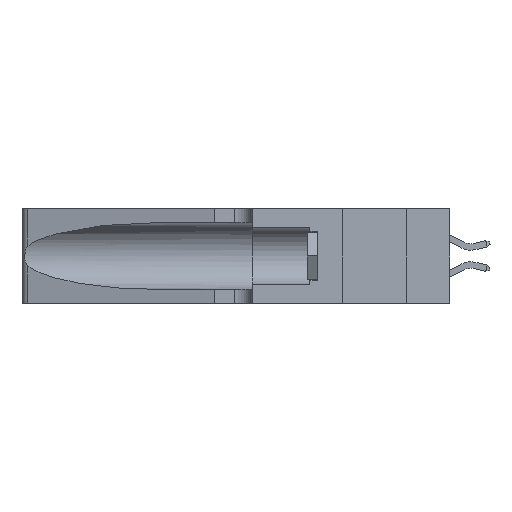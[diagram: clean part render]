
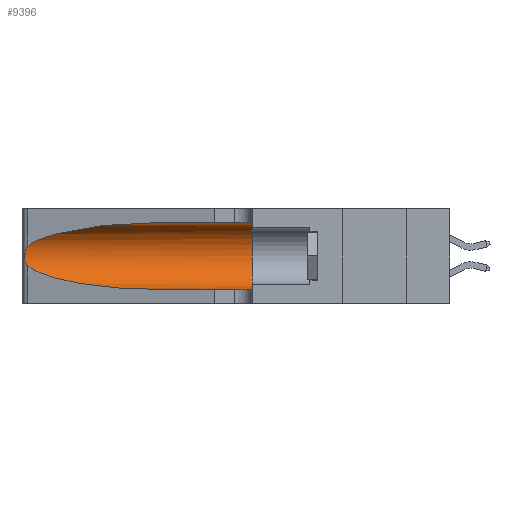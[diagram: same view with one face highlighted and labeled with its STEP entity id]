
A CAD part, left-side view. The second image highlights one B-rep face of the part: STEP entity #9396.
In plain terms, the highlighted cylindrical face has radius 3.308 mm (diameter 6.617 mm), a partial arc.
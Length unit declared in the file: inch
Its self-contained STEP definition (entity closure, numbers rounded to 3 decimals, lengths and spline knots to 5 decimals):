
#373 = CARTESIAN_POINT ( 'NONE',  ( 0.25487, 1.22718, 0.22369 ) ) ;
#752 = CARTESIAN_POINT ( 'NONE',  ( 0.18966, 0.96281, 0.05475 ) ) ;
#1265 =( BOUNDED_CURVE ( )  B_SPLINE_CURVE ( 3, ( #36432, #39600, #8391, #30260 ),
 .UNSPECIFIED., .F., .F. ) 
 B_SPLINE_CURVE_WITH_KNOTS ( ( 4, 4 ),
 ( 1.5708, 2.84003 ),
 .UNSPECIFIED. ) 
 CURVE ( )  GEOMETRIC_REPRESENTATION_ITEM ( )  RATIONAL_B_SPLINE_CURVE ( ( 1., 0.87, 0.87, 1. ) ) 
 REPRESENTATION_ITEM ( '' )  );
#2405 = VERTEX_POINT ( 'NONE', #38991 ) ;
#2751 = CARTESIAN_POINT ( 'NONE',  ( 0.26075, 1.23896, 0.178 ) ) ;
#2760 = VECTOR ( 'NONE', #14665, 39.37008 ) ;
#3657 = VERTEX_POINT ( 'NONE', #31638 ) ;
#3982 = VERTEX_POINT ( 'NONE', #23694 ) ;
#4009 = DIRECTION ( 'NONE',  ( 0., -1., 0. ) ) ;
#4351 = ORIENTED_EDGE ( 'NONE', *, *, #28018, .T. ) ;
#5039 = AXIS2_PLACEMENT_3D ( 'NONE', #30613, #11892, #33789 ) ;
#5984 = CARTESIAN_POINT ( 'NONE',  ( 0.25856, 1.23593, 0.16098 ) ) ;
#6492 = ORIENTED_EDGE ( 'NONE', *, *, #14828, .F. ) ;
#6604 = FACE_OUTER_BOUND ( 'NONE', #36968, .T. ) ;
#7046 = CARTESIAN_POINT ( 'NONE',  ( 0.2373, 1.15595, 0.08982 ) ) ;
#7260 = CARTESIAN_POINT ( 'NONE',  ( 0.1305, 1.61858, 0.185 ) ) ;
#7661 = ORIENTED_EDGE ( 'NONE', *, *, #28254, .T. ) ;
#8391 = CARTESIAN_POINT ( 'NONE',  ( 0.2373, 1.15595, 0.28018 ) ) ;
#8997 = CARTESIAN_POINT ( 'NONE',  ( 0.25487, 1.22718, 0.22369 ) ) ;
#9134 = CARTESIAN_POINT ( 'NONE',  ( 0.25639, 1.23186, 0.15144 ) ) ;
#9387 = CIRCLE ( 'NONE', #5039, 0.13025 ) ;
#9396 = ADVANCED_FACE ( 'NONE', ( #6604 ), #13944, .F. ) ;
#10197 = DIRECTION ( 'NONE',  ( 0., -1., 0. ) ) ;
#10382 = DIRECTION ( 'NONE',  ( 0., 0., -1. ) ) ;
#11090 = EDGE_CURVE ( 'NONE', #3982, #3657, #9387, .T. ) ;
#11173 = LINE ( 'NONE', #14266, #2760 ) ;
#11845 = VERTEX_POINT ( 'NONE', #34299 ) ;
#11892 = DIRECTION ( 'NONE',  ( 0., 1., 0. ) ) ;
#12264 = CARTESIAN_POINT ( 'NONE',  ( 0.25487, 1.22718, 0.14631 ) ) ;
#13944 = CYLINDRICAL_SURFACE ( 'NONE', #27838, 0.13025 ) ;
#14266 = CARTESIAN_POINT ( 'NONE',  ( 0.1305, 1.61858, 0.31525 ) ) ;
#14665 = DIRECTION ( 'NONE',  ( 0., -1., 0. ) ) ;
#14828 = EDGE_CURVE ( 'NONE', #2405, #3982, #11173, .T. ) ;
#15176 = VECTOR ( 'NONE', #10197, 39.37008 ) ;
#15287 = CARTESIAN_POINT ( 'NONE',  ( 0.25639, 1.23184, 0.21858 ) ) ;
#15944 =( BOUNDED_CURVE ( )  B_SPLINE_CURVE ( 3, ( #35210, #7046, #752, #22762 ),
 .UNSPECIFIED., .F., .T. ) 
 B_SPLINE_CURVE_WITH_KNOTS ( ( 4, 4 ),
 ( 3.44316, 4.71239 ),
 .UNSPECIFIED. ) 
 CURVE ( )  GEOMETRIC_REPRESENTATION_ITEM ( )  RATIONAL_B_SPLINE_CURVE ( ( 1., 0.87, 0.87, 1. ) ) 
 REPRESENTATION_ITEM ( '' )  );
#16809 = ORIENTED_EDGE ( 'NONE', *, *, #11090, .F. ) ;
#18411 = CARTESIAN_POINT ( 'NONE',  ( 0.25854, 1.2359, 0.20912 ) ) ;
#20166 = B_SPLINE_CURVE_WITH_KNOTS ( 'NONE', 3,
 ( #8997, #33899, #15287, #37200, #18411, #40346, #21565, #2751, #24719, #5984, #27876, #9134, #30989, #12264 ),
 .UNSPECIFIED., .F., .F.,
 ( 4, 2, 2, 2, 2, 2, 4 ),
 ( 0., 0.00027, 0.00053, 0.00107, 0.0016, 0.00187, 0.00214 ),
 .UNSPECIFIED. ) ;
#20733 = VERTEX_POINT ( 'NONE', #21870 ) ;
#21565 = CARTESIAN_POINT ( 'NONE',  ( 0.26075, 1.23896, 0.19203 ) ) ;
#21870 = CARTESIAN_POINT ( 'NONE',  ( 0.1305, 0.72297, 0.05475 ) ) ;
#22762 = CARTESIAN_POINT ( 'NONE',  ( 0.1305, 0.72297, 0.05475 ) ) ;
#23694 = CARTESIAN_POINT ( 'NONE',  ( 0.1305, 0.35, 0.31525 ) ) ;
#24719 = CARTESIAN_POINT ( 'NONE',  ( 0.26017, 1.23833, 0.17102 ) ) ;
#26783 = VERTEX_POINT ( 'NONE', #373 ) ;
#27407 = ORIENTED_EDGE ( 'NONE', *, *, #35561, .T. ) ;
#27838 = AXIS2_PLACEMENT_3D ( 'NONE', #7260, #4009, #10382 ) ;
#27876 = CARTESIAN_POINT ( 'NONE',  ( 0.25789, 1.23486, 0.15765 ) ) ;
#28018 = EDGE_CURVE ( 'NONE', #11845, #20733, #15944, .T. ) ;
#28254 = EDGE_CURVE ( 'NONE', #2405, #26783, #1265, .T. ) ;
#28414 = ORIENTED_EDGE ( 'NONE', *, *, #36589, .T. ) ;
#30260 = CARTESIAN_POINT ( 'NONE',  ( 0.25487, 1.22718, 0.22369 ) ) ;
#30613 = CARTESIAN_POINT ( 'NONE',  ( 0.1305, 0.35, 0.185 ) ) ;
#30989 = CARTESIAN_POINT ( 'NONE',  ( 0.25555, 1.22993, 0.14849 ) ) ;
#31638 = CARTESIAN_POINT ( 'NONE',  ( 0.1305, 0.35, 0.05475 ) ) ;
#33789 = DIRECTION ( 'NONE',  ( 0., 0., 1. ) ) ;
#33899 = CARTESIAN_POINT ( 'NONE',  ( 0.25555, 1.22994, 0.2215 ) ) ;
#34299 = CARTESIAN_POINT ( 'NONE',  ( 0.25487, 1.22718, 0.14631 ) ) ;
#35210 = CARTESIAN_POINT ( 'NONE',  ( 0.25487, 1.22718, 0.14631 ) ) ;
#35561 = EDGE_CURVE ( 'NONE', #20733, #3657, #40168, .T. ) ;
#36432 = CARTESIAN_POINT ( 'NONE',  ( 0.1305, 0.72297, 0.31525 ) ) ;
#36589 = EDGE_CURVE ( 'NONE', #26783, #11845, #20166, .T. ) ;
#36968 = EDGE_LOOP ( 'NONE', ( #7661, #28414, #4351, #27407, #16809, #6492 ) ) ;
#37200 = CARTESIAN_POINT ( 'NONE',  ( 0.25787, 1.23484, 0.2124 ) ) ;
#38260 = CARTESIAN_POINT ( 'NONE',  ( 0.1305, 1.61858, 0.05475 ) ) ;
#38991 = CARTESIAN_POINT ( 'NONE',  ( 0.1305, 0.72297, 0.31525 ) ) ;
#39600 = CARTESIAN_POINT ( 'NONE',  ( 0.18966, 0.96281, 0.31525 ) ) ;
#40168 = LINE ( 'NONE', #38260, #15176 ) ;
#40346 = CARTESIAN_POINT ( 'NONE',  ( 0.26018, 1.23835, 0.19895 ) ) ;
